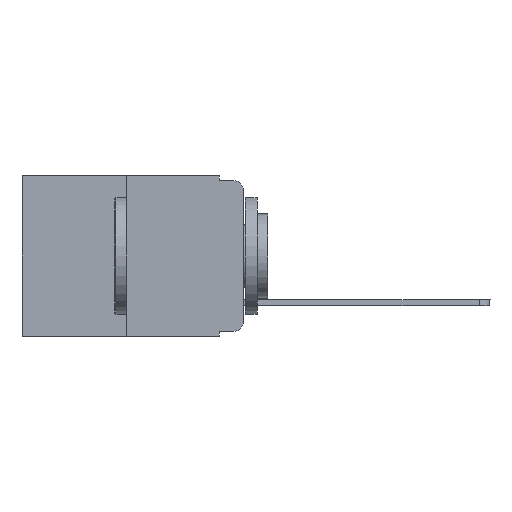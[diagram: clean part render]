
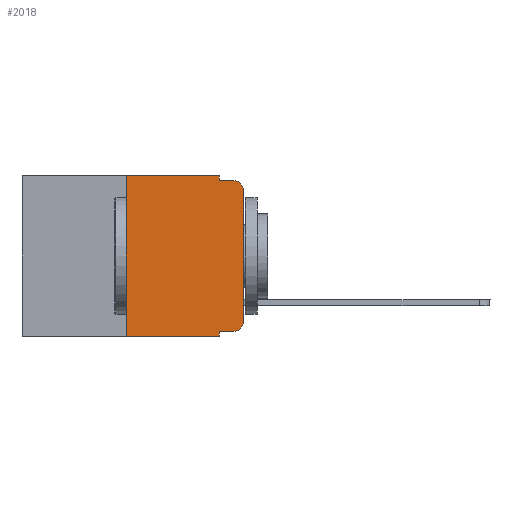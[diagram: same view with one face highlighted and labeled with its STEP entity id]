
A CAD part, left-side view. The second image highlights one B-rep face of the part: STEP entity #2018.
In plain terms, the highlighted planar face has unit normal (-1, 0, 0).
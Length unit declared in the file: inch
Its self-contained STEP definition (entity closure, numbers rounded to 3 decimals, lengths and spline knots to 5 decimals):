
#11 = LINE ( 'NONE', #6513, #9402 ) ;
#74 = EDGE_CURVE ( 'NONE', #6073, #8195, #10532, .T. ) ;
#773 = ORIENTED_EDGE ( 'NONE', *, *, #950, .F. ) ;
#903 = LINE ( 'NONE', #2783, #7641 ) ;
#920 = DIRECTION ( 'NONE',  ( 0., 0., -1. ) ) ;
#950 = EDGE_CURVE ( 'NONE', #5401, #11455, #9976, .T. ) ;
#992 = CARTESIAN_POINT ( 'NONE',  ( 0., 0.051, -0.333 ) ) ;
#1087 = CARTESIAN_POINT ( 'NONE',  ( 0., 0.02, -0.313 ) ) ;
#1172 = CARTESIAN_POINT ( 'NONE',  ( 0., 0.25, 0. ) ) ;
#1255 = ORIENTED_EDGE ( 'NONE', *, *, #74, .F. ) ;
#1288 = VERTEX_POINT ( 'NONE', #7632 ) ;
#1381 = VERTEX_POINT ( 'NONE', #10459 ) ;
#1521 = ORIENTED_EDGE ( 'NONE', *, *, #7993, .F. ) ;
#1576 = DIRECTION ( 'NONE',  ( 0., 0., -1. ) ) ;
#1639 = EDGE_CURVE ( 'NONE', #6279, #8766, #8178, .T. ) ;
#1832 = DIRECTION ( 'NONE',  ( 0., 0., 1. ) ) ;
#1918 = DIRECTION ( 'NONE',  ( 0., -1., 0. ) ) ;
#1948 = CIRCLE ( 'NONE', #8771, 0.02 ) ;
#2018 = ADVANCED_FACE ( 'NONE', ( #10990 ), #3468, .F. ) ;
#2092 = EDGE_CURVE ( 'NONE', #8766, #2541, #1948, .T. ) ;
#2493 = ORIENTED_EDGE ( 'NONE', *, *, #5428, .T. ) ;
#2537 = AXIS2_PLACEMENT_3D ( 'NONE', #10012, #11810, #1576 ) ;
#2541 = VERTEX_POINT ( 'NONE', #8368 ) ;
#2766 = ORIENTED_EDGE ( 'NONE', *, *, #8350, .T. ) ;
#2770 = LINE ( 'NONE', #8377, #8044 ) ;
#2783 = CARTESIAN_POINT ( 'NONE',  ( 0., 0.051, 0. ) ) ;
#3044 = ORIENTED_EDGE ( 'NONE', *, *, #6496, .F. ) ;
#3468 = PLANE ( 'NONE',  #2537 ) ;
#3472 = ORIENTED_EDGE ( 'NONE', *, *, #4318, .F. ) ;
#4032 = CARTESIAN_POINT ( 'NONE',  ( 0., 0.051, -0.343 ) ) ;
#4143 = EDGE_LOOP ( 'NONE', ( #7665, #9539, #3044, #773, #3472, #1255, #2766, #1521, #2493, #6215 ) ) ;
#4318 = EDGE_CURVE ( 'NONE', #8195, #5401, #11, .T. ) ;
#4434 = LINE ( 'NONE', #11747, #6151 ) ;
#4748 = DIRECTION ( 'NONE',  ( -1., 0., 0. ) ) ;
#4844 = CARTESIAN_POINT ( 'NONE',  ( 0., 0.051, 0. ) ) ;
#5401 = VERTEX_POINT ( 'NONE', #4844 ) ;
#5428 = EDGE_CURVE ( 'NONE', #1288, #1381, #5667, .T. ) ;
#5657 = CARTESIAN_POINT ( 'NONE',  ( 0., 0., -0.03 ) ) ;
#5667 = LINE ( 'NONE', #992, #6259 ) ;
#5918 = VECTOR ( 'NONE', #10398, 39.37008 ) ;
#6073 = VERTEX_POINT ( 'NONE', #7254 ) ;
#6151 = VECTOR ( 'NONE', #11051, 39.37008 ) ;
#6163 = DIRECTION ( 'NONE',  ( 0., 0., -1. ) ) ;
#6215 = ORIENTED_EDGE ( 'NONE', *, *, #7443, .T. ) ;
#6259 = VECTOR ( 'NONE', #9418, 39.37008 ) ;
#6279 = VERTEX_POINT ( 'NONE', #7674 ) ;
#6496 = EDGE_CURVE ( 'NONE', #11455, #2541, #4434, .T. ) ;
#6513 = CARTESIAN_POINT ( 'NONE',  ( 0., 0.473, 0. ) ) ;
#7201 = VERTEX_POINT ( 'NONE', #4032 ) ;
#7254 = CARTESIAN_POINT ( 'NONE',  ( 0., 0.25, -0.343 ) ) ;
#7348 = VECTOR ( 'NONE', #6163, 39.37008 ) ;
#7379 = CARTESIAN_POINT ( 'NONE',  ( 0., 0., 0. ) ) ;
#7443 = EDGE_CURVE ( 'NONE', #1381, #6279, #7527, .T. ) ;
#7527 = CIRCLE ( 'NONE', #9276, 0.02 ) ;
#7632 = CARTESIAN_POINT ( 'NONE',  ( 0., 0.051, -0.333 ) ) ;
#7641 = VECTOR ( 'NONE', #9441, 39.37008 ) ;
#7665 = ORIENTED_EDGE ( 'NONE', *, *, #1639, .T. ) ;
#7674 = CARTESIAN_POINT ( 'NONE',  ( 0., 0., -0.313 ) ) ;
#7982 = VECTOR ( 'NONE', #1832, 39.37008 ) ;
#7993 = EDGE_CURVE ( 'NONE', #1288, #7201, #903, .T. ) ;
#8044 = VECTOR ( 'NONE', #1918, 39.37008 ) ;
#8178 = LINE ( 'NONE', #7379, #7982 ) ;
#8195 = VERTEX_POINT ( 'NONE', #11795 ) ;
#8219 = CARTESIAN_POINT ( 'NONE',  ( 0., 0.02, -0.03 ) ) ;
#8350 = EDGE_CURVE ( 'NONE', #6073, #7201, #2770, .T. ) ;
#8368 = CARTESIAN_POINT ( 'NONE',  ( 0., 0.02, -0.01 ) ) ;
#8377 = CARTESIAN_POINT ( 'NONE',  ( 0., 0.473, -0.343 ) ) ;
#8766 = VERTEX_POINT ( 'NONE', #5657 ) ;
#8771 = AXIS2_PLACEMENT_3D ( 'NONE', #8219, #10074, #9090 ) ;
#9090 = DIRECTION ( 'NONE',  ( 0., 0., -1. ) ) ;
#9276 = AXIS2_PLACEMENT_3D ( 'NONE', #1087, #4748, #920 ) ;
#9338 = DIRECTION ( 'NONE',  ( 0., -1., 0. ) ) ;
#9402 = VECTOR ( 'NONE', #9338, 39.37008 ) ;
#9418 = DIRECTION ( 'NONE',  ( 0., -1., 0. ) ) ;
#9441 = DIRECTION ( 'NONE',  ( 0., 0., -1. ) ) ;
#9539 = ORIENTED_EDGE ( 'NONE', *, *, #2092, .T. ) ;
#9976 = LINE ( 'NONE', #10953, #7348 ) ;
#10012 = CARTESIAN_POINT ( 'NONE',  ( 0., 0.473, 0. ) ) ;
#10074 = DIRECTION ( 'NONE',  ( -1., 0., 0. ) ) ;
#10398 = DIRECTION ( 'NONE',  ( 0., 0., 1. ) ) ;
#10459 = CARTESIAN_POINT ( 'NONE',  ( 0., 0.02, -0.333 ) ) ;
#10532 = LINE ( 'NONE', #1172, #5918 ) ;
#10953 = CARTESIAN_POINT ( 'NONE',  ( 0., 0.051, 0. ) ) ;
#10990 = FACE_OUTER_BOUND ( 'NONE', #4143, .T. ) ;
#11051 = DIRECTION ( 'NONE',  ( 0., -1., 0. ) ) ;
#11455 = VERTEX_POINT ( 'NONE', #11982 ) ;
#11747 = CARTESIAN_POINT ( 'NONE',  ( 0., 0.051, -0.01 ) ) ;
#11795 = CARTESIAN_POINT ( 'NONE',  ( 0., 0.25, 0. ) ) ;
#11810 = DIRECTION ( 'NONE',  ( 1., 0., 0. ) ) ;
#11982 = CARTESIAN_POINT ( 'NONE',  ( 0., 0.051, -0.01 ) ) ;
